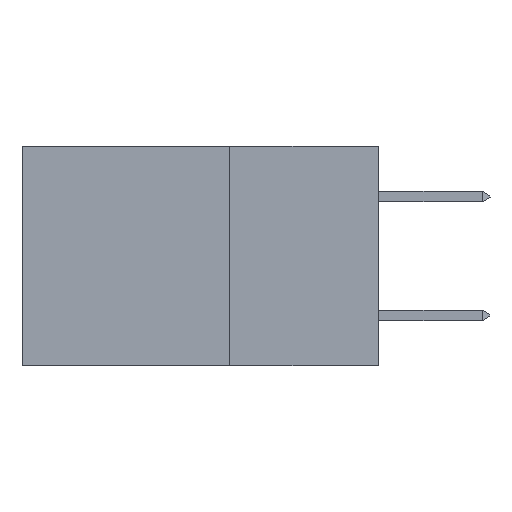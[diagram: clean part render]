
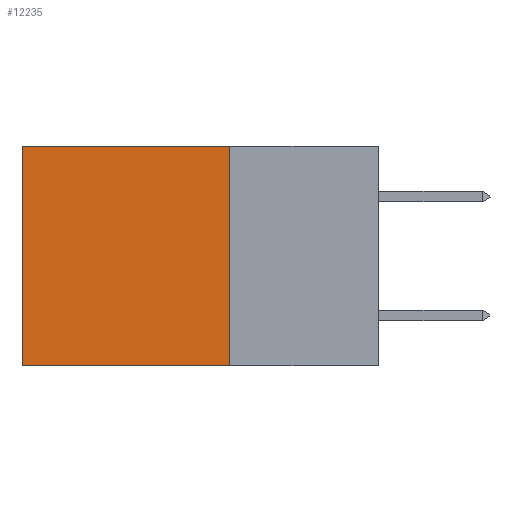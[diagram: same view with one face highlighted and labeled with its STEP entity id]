
A CAD part, left-side view. The second image highlights one B-rep face of the part: STEP entity #12235.
In plain terms, the highlighted planar face has unit normal (-1, 0, 0).
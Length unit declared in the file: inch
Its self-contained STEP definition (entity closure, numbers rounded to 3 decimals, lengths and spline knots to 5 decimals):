
#196 = FACE_OUTER_BOUND ( 'NONE', #21209, .T. ) ;
#335 = LINE ( 'NONE', #23030, #4645 ) ;
#2028 = VECTOR ( 'NONE', #15811, 39.37008 ) ;
#2781 = EDGE_CURVE ( 'NONE', #17671, #14884, #21715, .T. ) ;
#2960 = CARTESIAN_POINT ( 'NONE',  ( 0.298, 0.6, 0. ) ) ;
#3005 = LINE ( 'NONE', #2960, #17611 ) ;
#3731 = CARTESIAN_POINT ( 'NONE',  ( 0.298, 0.25, -0.37 ) ) ;
#4645 = VECTOR ( 'NONE', #12669, 39.37008 ) ;
#6585 = DIRECTION ( 'NONE',  ( 0., 1., 0. ) ) ;
#9062 = VERTEX_POINT ( 'NONE', #11683 ) ;
#9449 = ORIENTED_EDGE ( 'NONE', *, *, #24619, .T. ) ;
#10187 = CARTESIAN_POINT ( 'NONE',  ( 0.298, 0.6, -0.37 ) ) ;
#10612 = PLANE ( 'NONE',  #19544 ) ;
#11531 = CARTESIAN_POINT ( 'NONE',  ( 0.298, 0.25, 0. ) ) ;
#11683 = CARTESIAN_POINT ( 'NONE',  ( 0.298, 0.25, 0. ) ) ;
#12193 = VERTEX_POINT ( 'NONE', #23358 ) ;
#12235 = ADVANCED_FACE ( 'NONE', ( #196 ), #10612, .F. ) ;
#12330 = LINE ( 'NONE', #11531, #2028 ) ;
#12669 = DIRECTION ( 'NONE',  ( 0., 1., 0. ) ) ;
#13164 = CARTESIAN_POINT ( 'NONE',  ( 0.298, 0.25, -0.37 ) ) ;
#14884 = VERTEX_POINT ( 'NONE', #10187 ) ;
#14967 = ORIENTED_EDGE ( 'NONE', *, *, #15484, .T. ) ;
#15484 = EDGE_CURVE ( 'NONE', #12193, #14884, #3005, .T. ) ;
#15491 = EDGE_CURVE ( 'NONE', #9062, #17671, #12330, .T. ) ;
#15811 = DIRECTION ( 'NONE',  ( 0., 0., -1. ) ) ;
#16806 = DIRECTION ( 'NONE',  ( 0., 0., -1. ) ) ;
#17611 = VECTOR ( 'NONE', #22272, 39.37008 ) ;
#17671 = VERTEX_POINT ( 'NONE', #3731 ) ;
#18745 = VECTOR ( 'NONE', #6585, 39.37008 ) ;
#18760 = ORIENTED_EDGE ( 'NONE', *, *, #15491, .F. ) ;
#19544 = AXIS2_PLACEMENT_3D ( 'NONE', #25420, #22996, #16806 ) ;
#21209 = EDGE_LOOP ( 'NONE', ( #14967, #21397, #18760, #9449 ) ) ;
#21397 = ORIENTED_EDGE ( 'NONE', *, *, #2781, .F. ) ;
#21715 = LINE ( 'NONE', #13164, #18745 ) ;
#22272 = DIRECTION ( 'NONE',  ( 0., 0., -1. ) ) ;
#22996 = DIRECTION ( 'NONE',  ( 1., 0., 0. ) ) ;
#23030 = CARTESIAN_POINT ( 'NONE',  ( 0.298, 0.25, 0. ) ) ;
#23358 = CARTESIAN_POINT ( 'NONE',  ( 0.298, 0.6, 0. ) ) ;
#24619 = EDGE_CURVE ( 'NONE', #9062, #12193, #335, .T. ) ;
#25420 = CARTESIAN_POINT ( 'NONE',  ( 0.298, 0.25, 0. ) ) ;
